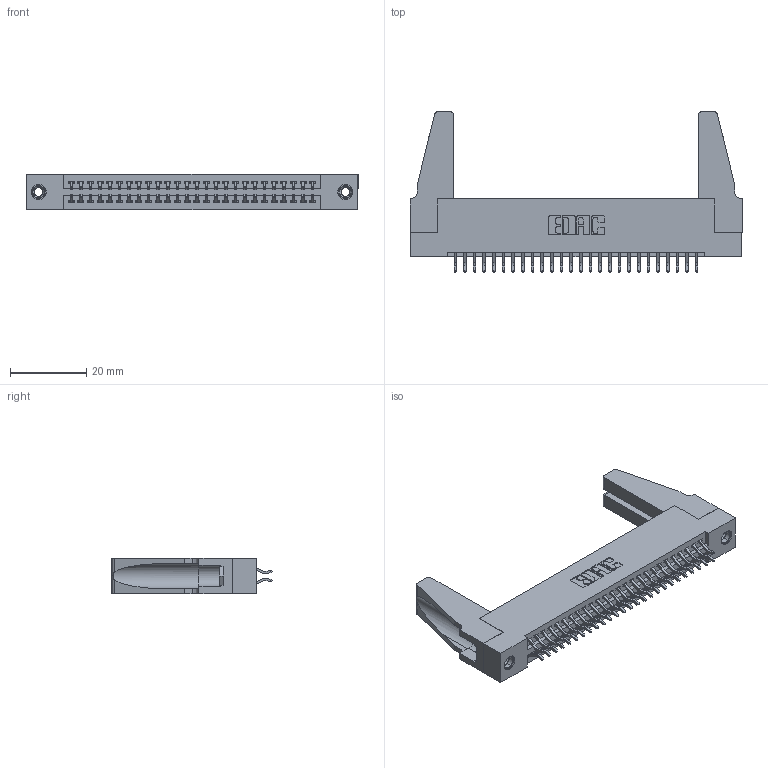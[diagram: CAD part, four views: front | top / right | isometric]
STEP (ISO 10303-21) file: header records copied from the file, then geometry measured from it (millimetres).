
FILE_DESCRIPTION (( 'STEP AP203' ), '1' );
FILE_NAME ('345-052-556-288.STEP', '2019-10-29T17:17:41', ( '' ), ( '' ), 'SwSTEP 2.0', 'SolidWorks 2016', '' );
FILE_SCHEMA (( 'CONFIG_CONTROL_DESIGN' ));
Length unit declared in the file: inch
Products named in the file (5): 345 Part_Flush Mounting Lugs - 0.156 Dia-TH; 345-220-078_345-220-088; 345-250-001_345-250-001-102; 345-052-556-288; 345-292-001_556 Tail
Assembly tree (57 placements, depth 2):
  345-052-556-288
    345 Part_Flush Mounting Lugs - 0.156 Dia-TH
    345-292-001_556 Tail  x52
    345-250-001_345-250-001-102  x2
    345-220-078_345-220-088  x2
Bounding box: 87.27 x 42.1 x 9.4 mm (x, y, z)
Volume: 11579.8 mm3; surface area: 15075.9 mm2
Topology: 57 solids, 57 shells, 3162 faces, 9339 edges, 6146 vertices
Faces by surface type: plane 2076, cylinder 1070, cone 12, torus 4
Entity records: 24922 total; most frequent: CARTESIAN_POINT 4202, ORIENTED_EDGE 4084, DIRECTION 3718, EDGE_CURVE 2042, LINE 1756, VECTOR 1756, VERTEX_POINT 1354, AXIS2_PLACEMENT_3D 981
